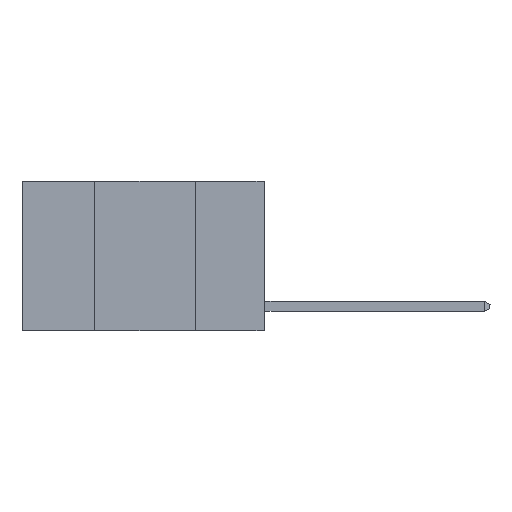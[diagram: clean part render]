
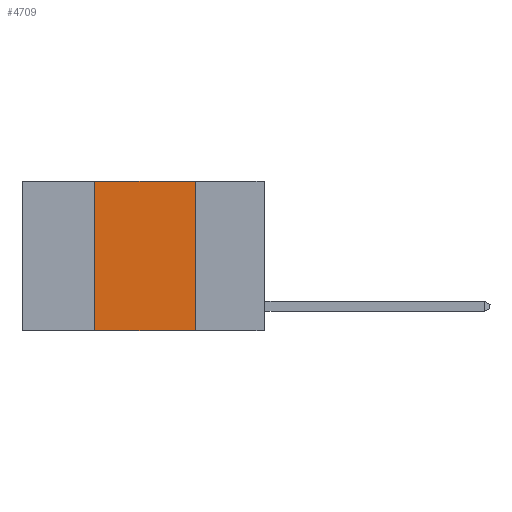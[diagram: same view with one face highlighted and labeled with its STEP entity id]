
A CAD part, left-side view. The second image highlights one B-rep face of the part: STEP entity #4709.
In plain terms, the highlighted planar face has unit normal (-1, 0, 0).
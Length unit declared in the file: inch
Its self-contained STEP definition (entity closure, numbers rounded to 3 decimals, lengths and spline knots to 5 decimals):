
#34 = CARTESIAN_POINT ( 'NONE',  ( 0., 0.6, 0. ) ) ;
#464 = ORIENTED_EDGE ( 'NONE', *, *, #19224, .F. ) ;
#848 = EDGE_LOOP ( 'NONE', ( #6807, #11419, #464, #8768 ) ) ;
#1419 = EDGE_CURVE ( 'NONE', #10990, #13780, #3703, .T. ) ;
#2078 = LINE ( 'NONE', #8949, #14537 ) ;
#2479 = VECTOR ( 'NONE', #13655, 39.37008 ) ;
#3405 = EDGE_CURVE ( 'NONE', #7274, #10990, #14895, .T. ) ;
#3508 = CARTESIAN_POINT ( 'NONE',  ( 0., 0.6, -0.37 ) ) ;
#3702 = VECTOR ( 'NONE', #7651, 39.37008 ) ;
#3703 = LINE ( 'NONE', #12030, #2479 ) ;
#3869 = EDGE_CURVE ( 'NONE', #19462, #13780, #12740, .T. ) ;
#4709 = ADVANCED_FACE ( 'NONE', ( #10200 ), #9967, .F. ) ;
#4771 = CARTESIAN_POINT ( 'NONE',  ( 0., 0.17, -0.37 ) ) ;
#5155 = DIRECTION ( 'NONE',  ( 0., -1., 0. ) ) ;
#6807 = ORIENTED_EDGE ( 'NONE', *, *, #1419, .F. ) ;
#7274 = VERTEX_POINT ( 'NONE', #13958 ) ;
#7279 = DIRECTION ( 'NONE',  ( 0., 0., 1. ) ) ;
#7651 = DIRECTION ( 'NONE',  ( 0., -1., 0. ) ) ;
#8768 = ORIENTED_EDGE ( 'NONE', *, *, #3869, .T. ) ;
#8949 = CARTESIAN_POINT ( 'NONE',  ( 0., 0.42, 0. ) ) ;
#9967 = PLANE ( 'NONE',  #15937 ) ;
#10200 = FACE_OUTER_BOUND ( 'NONE', #848, .T. ) ;
#10752 = VECTOR ( 'NONE', #5155, 39.37008 ) ;
#10990 = VERTEX_POINT ( 'NONE', #18633 ) ;
#11419 = ORIENTED_EDGE ( 'NONE', *, *, #3405, .F. ) ;
#11849 = CARTESIAN_POINT ( 'NONE',  ( 0., 0.42, -0.37 ) ) ;
#12030 = CARTESIAN_POINT ( 'NONE',  ( 0., 0.17, 0. ) ) ;
#12740 = LINE ( 'NONE', #3508, #10752 ) ;
#13004 = CARTESIAN_POINT ( 'NONE',  ( 0., 0.6, 0. ) ) ;
#13199 = DIRECTION ( 'NONE',  ( 0., 0., -1. ) ) ;
#13655 = DIRECTION ( 'NONE',  ( 0., 0., -1. ) ) ;
#13780 = VERTEX_POINT ( 'NONE', #4771 ) ;
#13958 = CARTESIAN_POINT ( 'NONE',  ( 0., 0.42, 0. ) ) ;
#14537 = VECTOR ( 'NONE', #7279, 39.37008 ) ;
#14895 = LINE ( 'NONE', #34, #3702 ) ;
#15937 = AXIS2_PLACEMENT_3D ( 'NONE', #13004, #19326, #13199 ) ;
#18633 = CARTESIAN_POINT ( 'NONE',  ( 0., 0.17, 0. ) ) ;
#19224 = EDGE_CURVE ( 'NONE', #19462, #7274, #2078, .T. ) ;
#19326 = DIRECTION ( 'NONE',  ( 1., 0., 0. ) ) ;
#19462 = VERTEX_POINT ( 'NONE', #11849 ) ;
